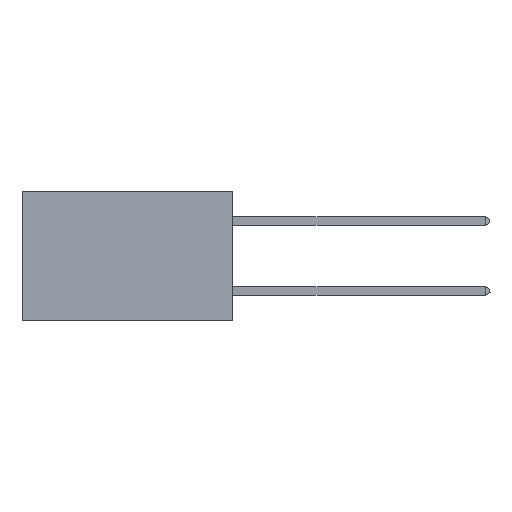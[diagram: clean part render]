
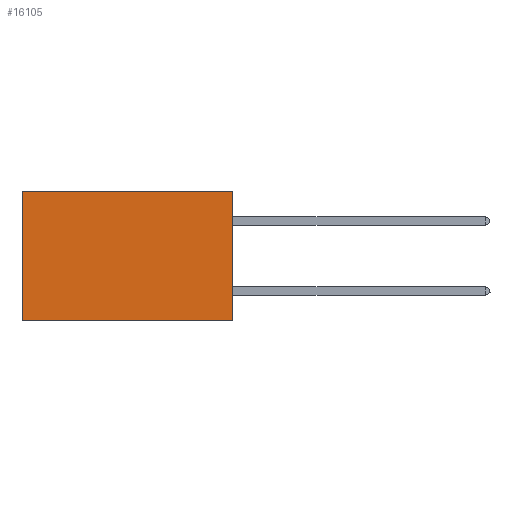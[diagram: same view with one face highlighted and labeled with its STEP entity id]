
A CAD part, left-side view. The second image highlights one B-rep face of the part: STEP entity #16105.
In plain terms, the highlighted planar face has unit normal (-1, 0, 0).
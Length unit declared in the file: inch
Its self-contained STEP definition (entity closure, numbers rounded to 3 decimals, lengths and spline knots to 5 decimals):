
#397 = ORIENTED_EDGE ( 'NONE', *, *, #13911, .F. ) ;
#789 = DIRECTION ( 'NONE',  ( 0., 0., -1. ) ) ;
#1529 = CARTESIAN_POINT ( 'NONE',  ( 0.2875, 0., 0. ) ) ;
#2079 = LINE ( 'NONE', #7185, #13199 ) ;
#3239 = LINE ( 'NONE', #15861, #9840 ) ;
#3264 = VERTEX_POINT ( 'NONE', #10563 ) ;
#3863 = VERTEX_POINT ( 'NONE', #26407 ) ;
#7185 = CARTESIAN_POINT ( 'NONE',  ( 0.2875, 0.6, 0. ) ) ;
#7707 = EDGE_LOOP ( 'NONE', ( #10300, #397, #14198, #13931 ) ) ;
#8058 = VERTEX_POINT ( 'NONE', #1529 ) ;
#9840 = VECTOR ( 'NONE', #11474, 39.37008 ) ;
#10195 = CARTESIAN_POINT ( 'NONE',  ( 0.2875, 0., -0.37 ) ) ;
#10196 = DIRECTION ( 'NONE',  ( 1., 0., 0. ) ) ;
#10300 = ORIENTED_EDGE ( 'NONE', *, *, #20589, .T. ) ;
#10563 = CARTESIAN_POINT ( 'NONE',  ( 0.2875, 0.6, -0.37 ) ) ;
#11474 = DIRECTION ( 'NONE',  ( 0., 1., 0. ) ) ;
#12237 = CARTESIAN_POINT ( 'NONE',  ( 0.2875, 0., 0. ) ) ;
#13199 = VECTOR ( 'NONE', #13896, 39.37008 ) ;
#13896 = DIRECTION ( 'NONE',  ( 0., 0., -1. ) ) ;
#13911 = EDGE_CURVE ( 'NONE', #24130, #3264, #3239, .T. ) ;
#13931 = ORIENTED_EDGE ( 'NONE', *, *, #20883, .T. ) ;
#14198 = ORIENTED_EDGE ( 'NONE', *, *, #16673, .F. ) ;
#14398 = CARTESIAN_POINT ( 'NONE',  ( 0.2875, 0., 0. ) ) ;
#14902 = LINE ( 'NONE', #25554, #15980 ) ;
#15626 = VECTOR ( 'NONE', #789, 39.37008 ) ;
#15861 = CARTESIAN_POINT ( 'NONE',  ( 0.2875, 0., -0.37 ) ) ;
#15980 = VECTOR ( 'NONE', #23672, 39.37008 ) ;
#16105 = ADVANCED_FACE ( 'NONE', ( #28155 ), #16527, .F. ) ;
#16527 = PLANE ( 'NONE',  #17159 ) ;
#16673 = EDGE_CURVE ( 'NONE', #8058, #24130, #20841, .T. ) ;
#17159 = AXIS2_PLACEMENT_3D ( 'NONE', #14398, #10196, #25369 ) ;
#20589 = EDGE_CURVE ( 'NONE', #3863, #3264, #2079, .T. ) ;
#20841 = LINE ( 'NONE', #12237, #15626 ) ;
#20883 = EDGE_CURVE ( 'NONE', #8058, #3863, #14902, .T. ) ;
#23672 = DIRECTION ( 'NONE',  ( 0., 1., 0. ) ) ;
#24130 = VERTEX_POINT ( 'NONE', #10195 ) ;
#25369 = DIRECTION ( 'NONE',  ( 0., 0., -1. ) ) ;
#25554 = CARTESIAN_POINT ( 'NONE',  ( 0.2875, 0., 0. ) ) ;
#26407 = CARTESIAN_POINT ( 'NONE',  ( 0.2875, 0.6, 0. ) ) ;
#28155 = FACE_OUTER_BOUND ( 'NONE', #7707, .T. ) ;
